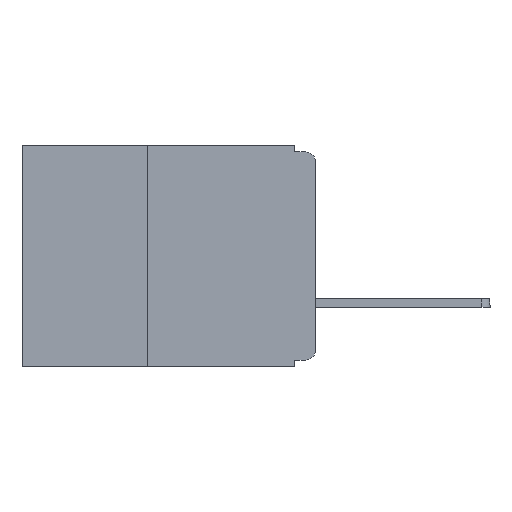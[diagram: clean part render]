
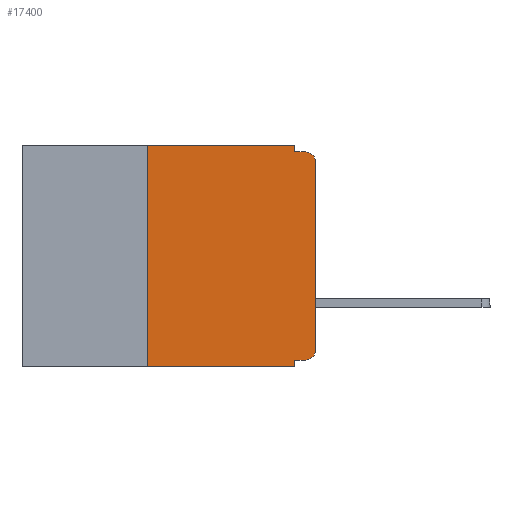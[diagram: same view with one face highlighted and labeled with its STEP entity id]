
A CAD part, left-side view. The second image highlights one B-rep face of the part: STEP entity #17400.
In plain terms, the highlighted planar face has unit normal (-1, 0, 0).
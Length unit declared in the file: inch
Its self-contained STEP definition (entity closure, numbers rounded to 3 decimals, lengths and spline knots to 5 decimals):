
#712 = VERTEX_POINT ( 'NONE', #24475 ) ;
#884 = CARTESIAN_POINT ( 'NONE',  ( 0., 0.031, 0. ) ) ;
#1041 = ORIENTED_EDGE ( 'NONE', *, *, #1765, .F. ) ;
#1171 = DIRECTION ( 'NONE',  ( 1., 0., 0. ) ) ;
#1523 = CARTESIAN_POINT ( 'NONE',  ( 0., 0., -0.01 ) ) ;
#1765 = EDGE_CURVE ( 'NONE', #2703, #15529, #15090, .T. ) ;
#1804 = VECTOR ( 'NONE', #15196, 39.37008 ) ;
#1877 = CARTESIAN_POINT ( 'NONE',  ( 0., 0.015, -0.01 ) ) ;
#1954 = CARTESIAN_POINT ( 'NONE',  ( 0., 0.031, -0.33 ) ) ;
#2440 = ORIENTED_EDGE ( 'NONE', *, *, #6746, .F. ) ;
#2446 = LINE ( 'NONE', #884, #22027 ) ;
#2703 = VERTEX_POINT ( 'NONE', #22214 ) ;
#2814 = ORIENTED_EDGE ( 'NONE', *, *, #15783, .F. ) ;
#2819 = DIRECTION ( 'NONE',  ( 0., 0., -1. ) ) ;
#2825 = VECTOR ( 'NONE', #3886, 39.37008 ) ;
#2858 = VERTEX_POINT ( 'NONE', #1877 ) ;
#2985 = CARTESIAN_POINT ( 'NONE',  ( 0., 0.015, -0.305 ) ) ;
#3227 = ORIENTED_EDGE ( 'NONE', *, *, #18432, .T. ) ;
#3886 = DIRECTION ( 'NONE',  ( 0., 0., -1. ) ) ;
#3891 = CARTESIAN_POINT ( 'NONE',  ( 0., 0., -0.32 ) ) ;
#4900 = DIRECTION ( 'NONE',  ( 0., 0., -1. ) ) ;
#4925 = PLANE ( 'NONE',  #7528 ) ;
#5043 = AXIS2_PLACEMENT_3D ( 'NONE', #9096, #22389, #11015 ) ;
#5057 = ORIENTED_EDGE ( 'NONE', *, *, #7194, .F. ) ;
#5803 = CARTESIAN_POINT ( 'NONE',  ( 0., 0.25, -0.33 ) ) ;
#5863 = LINE ( 'NONE', #5803, #15313 ) ;
#6641 = VECTOR ( 'NONE', #22336, 39.37008 ) ;
#6746 = EDGE_CURVE ( 'NONE', #7357, #712, #17294, .T. ) ;
#7168 = EDGE_LOOP ( 'NONE', ( #24026, #14952, #5057, #2814, #1041, #11299, #3227, #2440, #11107, #18425 ) ) ;
#7194 = EDGE_CURVE ( 'NONE', #24095, #2858, #11662, .T. ) ;
#7357 = VERTEX_POINT ( 'NONE', #9602 ) ;
#7528 = AXIS2_PLACEMENT_3D ( 'NONE', #23852, #1171, #14429 ) ;
#8680 = EDGE_CURVE ( 'NONE', #12624, #7357, #21980, .T. ) ;
#9096 = CARTESIAN_POINT ( 'NONE',  ( 0., 0.015, -0.025 ) ) ;
#9602 = CARTESIAN_POINT ( 'NONE',  ( 0., 0.031, -0.32 ) ) ;
#9765 = CARTESIAN_POINT ( 'NONE',  ( 0., 0.015, -0.32 ) ) ;
#9839 = EDGE_CURVE ( 'NONE', #15037, #2858, #14200, .T. ) ;
#10106 = CARTESIAN_POINT ( 'NONE',  ( 0., 0., -0.025 ) ) ;
#11015 = DIRECTION ( 'NONE',  ( 0., 0., -1. ) ) ;
#11107 = ORIENTED_EDGE ( 'NONE', *, *, #8680, .F. ) ;
#11264 = CARTESIAN_POINT ( 'NONE',  ( 0., 0., 0. ) ) ;
#11299 = ORIENTED_EDGE ( 'NONE', *, *, #23819, .F. ) ;
#11591 = EDGE_CURVE ( 'NONE', #12624, #22217, #19237, .T. ) ;
#11662 = LINE ( 'NONE', #1523, #6641 ) ;
#12208 = VERTEX_POINT ( 'NONE', #19928 ) ;
#12336 = AXIS2_PLACEMENT_3D ( 'NONE', #2985, #16197, #4900 ) ;
#12344 = LINE ( 'NONE', #23152, #21833 ) ;
#12624 = VERTEX_POINT ( 'NONE', #9765 ) ;
#13433 = CARTESIAN_POINT ( 'NONE',  ( 0., 0.031, 0. ) ) ;
#13702 = DIRECTION ( 'NONE',  ( 0., -1., 0. ) ) ;
#14200 = CIRCLE ( 'NONE', #5043, 0.015 ) ;
#14429 = DIRECTION ( 'NONE',  ( 0., 0., -1. ) ) ;
#14872 = VECTOR ( 'NONE', #18855, 39.37008 ) ;
#14952 = ORIENTED_EDGE ( 'NONE', *, *, #9839, .T. ) ;
#15037 = VERTEX_POINT ( 'NONE', #10106 ) ;
#15090 = LINE ( 'NONE', #22797, #19546 ) ;
#15196 = DIRECTION ( 'NONE',  ( 0., 1., 0. ) ) ;
#15313 = VECTOR ( 'NONE', #17096, 39.37008 ) ;
#15343 = FACE_OUTER_BOUND ( 'NONE', #7168, .T. ) ;
#15431 = EDGE_CURVE ( 'NONE', #22217, #15037, #20531, .T. ) ;
#15529 = VERTEX_POINT ( 'NONE', #13433 ) ;
#15783 = EDGE_CURVE ( 'NONE', #15529, #24095, #2446, .T. ) ;
#16197 = DIRECTION ( 'NONE',  ( -1., 0., 0. ) ) ;
#16366 = CARTESIAN_POINT ( 'NONE',  ( 0., 0., -0.305 ) ) ;
#17096 = DIRECTION ( 'NONE',  ( 0., 0., 1. ) ) ;
#17294 = LINE ( 'NONE', #1954, #2825 ) ;
#17400 = ADVANCED_FACE ( 'NONE', ( #15343 ), #4925, .F. ) ;
#18425 = ORIENTED_EDGE ( 'NONE', *, *, #11591, .T. ) ;
#18432 = EDGE_CURVE ( 'NONE', #12208, #712, #12344, .T. ) ;
#18855 = DIRECTION ( 'NONE',  ( 0., 0., 1. ) ) ;
#19237 = CIRCLE ( 'NONE', #12336, 0.015 ) ;
#19546 = VECTOR ( 'NONE', #21835, 39.37008 ) ;
#19928 = CARTESIAN_POINT ( 'NONE',  ( 0., 0.25, -0.33 ) ) ;
#19949 = CARTESIAN_POINT ( 'NONE',  ( 0., 0.031, -0.01 ) ) ;
#20531 = LINE ( 'NONE', #11264, #14872 ) ;
#21833 = VECTOR ( 'NONE', #13702, 39.37008 ) ;
#21835 = DIRECTION ( 'NONE',  ( 0., -1., 0. ) ) ;
#21980 = LINE ( 'NONE', #3891, #1804 ) ;
#22027 = VECTOR ( 'NONE', #2819, 39.37008 ) ;
#22214 = CARTESIAN_POINT ( 'NONE',  ( 0., 0.25, 0. ) ) ;
#22217 = VERTEX_POINT ( 'NONE', #16366 ) ;
#22336 = DIRECTION ( 'NONE',  ( 0., -1., 0. ) ) ;
#22389 = DIRECTION ( 'NONE',  ( -1., 0., 0. ) ) ;
#22797 = CARTESIAN_POINT ( 'NONE',  ( 0., 0.437, 0. ) ) ;
#23152 = CARTESIAN_POINT ( 'NONE',  ( 0., 0.437, -0.33 ) ) ;
#23819 = EDGE_CURVE ( 'NONE', #12208, #2703, #5863, .T. ) ;
#23852 = CARTESIAN_POINT ( 'NONE',  ( 0., 0.437, 0. ) ) ;
#24026 = ORIENTED_EDGE ( 'NONE', *, *, #15431, .T. ) ;
#24095 = VERTEX_POINT ( 'NONE', #19949 ) ;
#24475 = CARTESIAN_POINT ( 'NONE',  ( 0., 0.031, -0.33 ) ) ;
